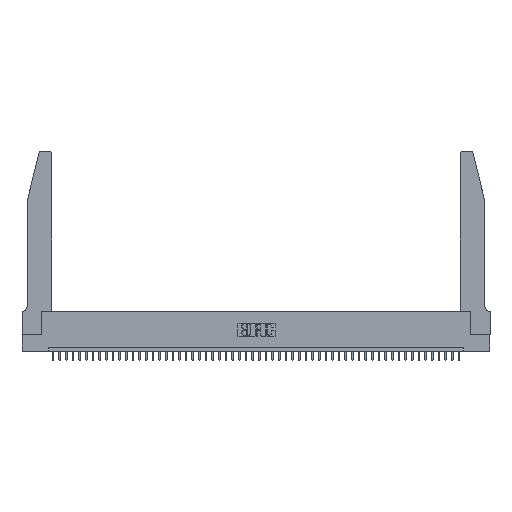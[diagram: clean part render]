
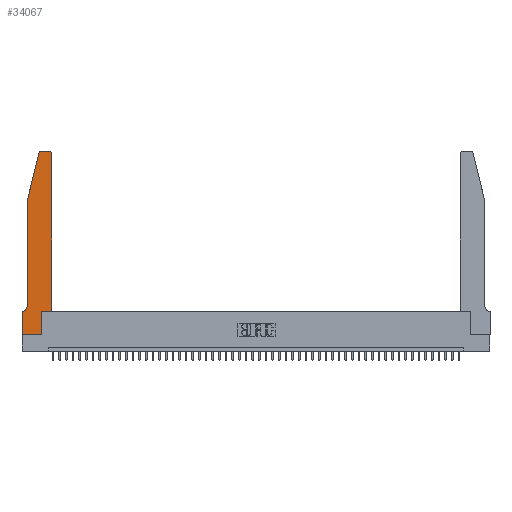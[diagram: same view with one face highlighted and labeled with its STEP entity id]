
A CAD part, top view. The second image highlights one B-rep face of the part: STEP entity #34067.
In plain terms, the highlighted planar face has unit normal (0, 0, 1).
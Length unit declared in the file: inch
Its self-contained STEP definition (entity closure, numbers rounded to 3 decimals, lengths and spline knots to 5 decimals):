
#1325 = CARTESIAN_POINT ( 'NONE',  ( 0.2865, 0., 0.37 ) ) ;
#2206 = CIRCLE ( 'NONE', #26130, 0.03 ) ;
#2451 = LINE ( 'NONE', #4916, #41391 ) ;
#2718 = CARTESIAN_POINT ( 'NONE',  ( 0.4505, 2.72, 0.37 ) ) ;
#3604 = ORIENTED_EDGE ( 'NONE', *, *, #19336, .T. ) ;
#4502 = VERTEX_POINT ( 'NONE', #13193 ) ;
#4597 = EDGE_CURVE ( 'NONE', #9620, #34337, #2451, .T. ) ;
#4763 = CARTESIAN_POINT ( 'NONE',  ( 0.0755, 2., 0.37 ) ) ;
#4907 = CARTESIAN_POINT ( 'NONE',  ( 0.2865, 0.35, 0.37 ) ) ;
#4916 = CARTESIAN_POINT ( 'NONE',  ( 0., 0., 0.37 ) ) ;
#5678 = VECTOR ( 'NONE', #31590, 39.37008 ) ;
#7504 = DIRECTION ( 'NONE',  ( 0., -1., 0. ) ) ;
#7708 = VECTOR ( 'NONE', #38015, 39.37008 ) ;
#8330 = DIRECTION ( 'NONE',  ( 1., 0., 0. ) ) ;
#8528 = ORIENTED_EDGE ( 'NONE', *, *, #44146, .T. ) ;
#9620 = VERTEX_POINT ( 'NONE', #20253 ) ;
#9783 = CARTESIAN_POINT ( 'NONE',  ( 0.284, 2.72, 0.37 ) ) ;
#10113 = DIRECTION ( 'NONE',  ( 0., 0., -1. ) ) ;
#10259 = CARTESIAN_POINT ( 'NONE',  ( 0.284, 2.75, 0.37 ) ) ;
#10966 = CARTESIAN_POINT ( 'NONE',  ( 0.0755, 2., 0.37 ) ) ;
#11324 = EDGE_CURVE ( 'NONE', #18200, #11853, #12774, .T. ) ;
#11853 = VERTEX_POINT ( 'NONE', #47703 ) ;
#12774 = LINE ( 'NONE', #24316, #5678 ) ;
#13193 = CARTESIAN_POINT ( 'NONE',  ( 0.0755, 2., 0.37 ) ) ;
#14984 = LINE ( 'NONE', #4907, #31451 ) ;
#15535 = DIRECTION ( 'NONE',  ( 1., 0., 0. ) ) ;
#17215 = VERTEX_POINT ( 'NONE', #43992 ) ;
#17474 = EDGE_CURVE ( 'NONE', #24694, #27683, #2206, .T. ) ;
#18200 = VERTEX_POINT ( 'NONE', #24591 ) ;
#19336 = EDGE_CURVE ( 'NONE', #4502, #25867, #27168, .T. ) ;
#20253 = CARTESIAN_POINT ( 'NONE',  ( 0., 0., 0.37 ) ) ;
#20793 = CARTESIAN_POINT ( 'NONE',  ( 0., 0., 0.37 ) ) ;
#21661 = EDGE_LOOP ( 'NONE', ( #42188, #37700, #41186, #3604, #47520, #36568, #32247, #37879, #8528, #22110, #46204, #23871 ) ) ;
#21702 = DIRECTION ( 'NONE',  ( 1., 0., 0. ) ) ;
#22110 = ORIENTED_EDGE ( 'NONE', *, *, #38982, .T. ) ;
#23223 = CARTESIAN_POINT ( 'NONE',  ( 0.4205, 2.75, 0.37 ) ) ;
#23714 = FACE_OUTER_BOUND ( 'NONE', #21661, .T. ) ;
#23871 = ORIENTED_EDGE ( 'NONE', *, *, #35837, .T. ) ;
#24080 = DIRECTION ( 'NONE',  ( 0., -1., 0. ) ) ;
#24316 = CARTESIAN_POINT ( 'NONE',  ( 0.0755, 0.35, 0.37 ) ) ;
#24438 = LINE ( 'NONE', #10966, #35706 ) ;
#24591 = CARTESIAN_POINT ( 'NONE',  ( 0.0055, 0.35, 0.37 ) ) ;
#24694 = VERTEX_POINT ( 'NONE', #10259 ) ;
#24720 = AXIS2_PLACEMENT_3D ( 'NONE', #40900, #36958, #21702 ) ;
#24932 = VECTOR ( 'NONE', #48756, 39.37008 ) ;
#25839 = CARTESIAN_POINT ( 'NONE',  ( 0.4505, 0.35, 0.37 ) ) ;
#25867 = VERTEX_POINT ( 'NONE', #36968 ) ;
#26130 = AXIS2_PLACEMENT_3D ( 'NONE', #9783, #45396, #15535 ) ;
#26341 = EDGE_CURVE ( 'NONE', #25867, #18200, #31864, .T. ) ;
#27168 = LINE ( 'NONE', #4763, #35510 ) ;
#27556 = AXIS2_PLACEMENT_3D ( 'NONE', #33810, #37622, #45180 ) ;
#27683 = VERTEX_POINT ( 'NONE', #33736 ) ;
#28768 = PLANE ( 'NONE',  #24720 ) ;
#28796 = LINE ( 'NONE', #34179, #34789 ) ;
#30575 = VECTOR ( 'NONE', #24080, 39.37008 ) ;
#31344 = EDGE_CURVE ( 'NONE', #11853, #9620, #45929, .T. ) ;
#31451 = VECTOR ( 'NONE', #35879, 39.37008 ) ;
#31590 = DIRECTION ( 'NONE',  ( -1., 0., 0. ) ) ;
#31864 = CIRCLE ( 'NONE', #35278, 0.07 ) ;
#32091 = VERTEX_POINT ( 'NONE', #25839 ) ;
#32247 = ORIENTED_EDGE ( 'NONE', *, *, #31344, .T. ) ;
#32684 = CARTESIAN_POINT ( 'NONE',  ( 0.0055, 0.42, 0.37 ) ) ;
#32842 = VERTEX_POINT ( 'NONE', #23223 ) ;
#33736 = CARTESIAN_POINT ( 'NONE',  ( 0.25487, 2.72718, 0.37 ) ) ;
#33810 = CARTESIAN_POINT ( 'NONE',  ( 0.4205, 2.72, 0.37 ) ) ;
#33878 = DIRECTION ( 'NONE',  ( -0.239, -0.971, 0. ) ) ;
#34067 = ADVANCED_FACE ( 'NONE', ( #23714 ), #28768, .T. ) ;
#34179 = CARTESIAN_POINT ( 'NONE',  ( 0.4505, 0.35, 0.37 ) ) ;
#34337 = VERTEX_POINT ( 'NONE', #1325 ) ;
#34789 = VECTOR ( 'NONE', #45551, 39.37008 ) ;
#35278 = AXIS2_PLACEMENT_3D ( 'NONE', #32684, #10113, #44096 ) ;
#35468 = LINE ( 'NONE', #41481, #7708 ) ;
#35510 = VECTOR ( 'NONE', #7504, 39.37008 ) ;
#35706 = VECTOR ( 'NONE', #33878, 39.37008 ) ;
#35837 = EDGE_CURVE ( 'NONE', #42768, #32842, #45995, .T. ) ;
#35879 = DIRECTION ( 'NONE',  ( 0., 1., 0. ) ) ;
#36568 = ORIENTED_EDGE ( 'NONE', *, *, #11324, .T. ) ;
#36958 = DIRECTION ( 'NONE',  ( 0., 0., 1. ) ) ;
#36968 = CARTESIAN_POINT ( 'NONE',  ( 0.0755, 0.42, 0.37 ) ) ;
#37399 = LINE ( 'NONE', #44677, #24932 ) ;
#37622 = DIRECTION ( 'NONE',  ( 0., 0., 1. ) ) ;
#37700 = ORIENTED_EDGE ( 'NONE', *, *, #17474, .T. ) ;
#37879 = ORIENTED_EDGE ( 'NONE', *, *, #4597, .T. ) ;
#38015 = DIRECTION ( 'NONE',  ( 0., 1., 0. ) ) ;
#38982 = EDGE_CURVE ( 'NONE', #17215, #32091, #28796, .T. ) ;
#40900 = CARTESIAN_POINT ( 'NONE',  ( 0., 0.35, 0.37 ) ) ;
#41186 = ORIENTED_EDGE ( 'NONE', *, *, #46406, .T. ) ;
#41391 = VECTOR ( 'NONE', #8330, 39.37008 ) ;
#41481 = CARTESIAN_POINT ( 'NONE',  ( 0.4505, 0.35, 0.37 ) ) ;
#41663 = EDGE_CURVE ( 'NONE', #32091, #42768, #35468, .T. ) ;
#42188 = ORIENTED_EDGE ( 'NONE', *, *, #44563, .T. ) ;
#42768 = VERTEX_POINT ( 'NONE', #2718 ) ;
#43992 = CARTESIAN_POINT ( 'NONE',  ( 0.2865, 0.35, 0.37 ) ) ;
#44096 = DIRECTION ( 'NONE',  ( -1., 0., 0. ) ) ;
#44146 = EDGE_CURVE ( 'NONE', #34337, #17215, #14984, .T. ) ;
#44563 = EDGE_CURVE ( 'NONE', #32842, #24694, #37399, .T. ) ;
#44677 = CARTESIAN_POINT ( 'NONE',  ( 0.2605, 2.75, 0.37 ) ) ;
#45180 = DIRECTION ( 'NONE',  ( 1., 0., 0. ) ) ;
#45396 = DIRECTION ( 'NONE',  ( 0., 0., 1. ) ) ;
#45551 = DIRECTION ( 'NONE',  ( 1., 0., 0. ) ) ;
#45929 = LINE ( 'NONE', #20793, #30575 ) ;
#45995 = CIRCLE ( 'NONE', #27556, 0.03 ) ;
#46204 = ORIENTED_EDGE ( 'NONE', *, *, #41663, .T. ) ;
#46406 = EDGE_CURVE ( 'NONE', #27683, #4502, #24438, .T. ) ;
#47520 = ORIENTED_EDGE ( 'NONE', *, *, #26341, .T. ) ;
#47703 = CARTESIAN_POINT ( 'NONE',  ( 0., 0.35, 0.37 ) ) ;
#48756 = DIRECTION ( 'NONE',  ( -1., 0., 0. ) ) ;
